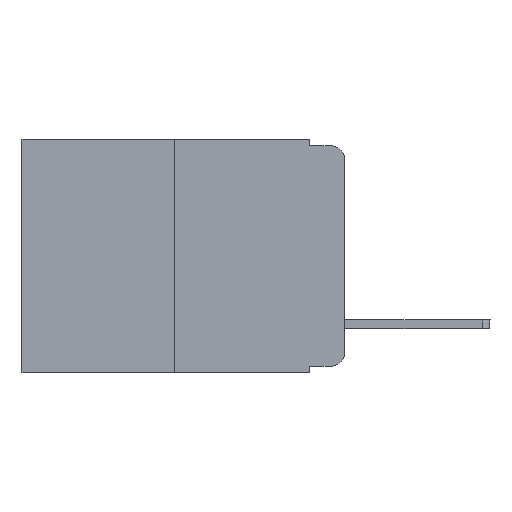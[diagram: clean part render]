
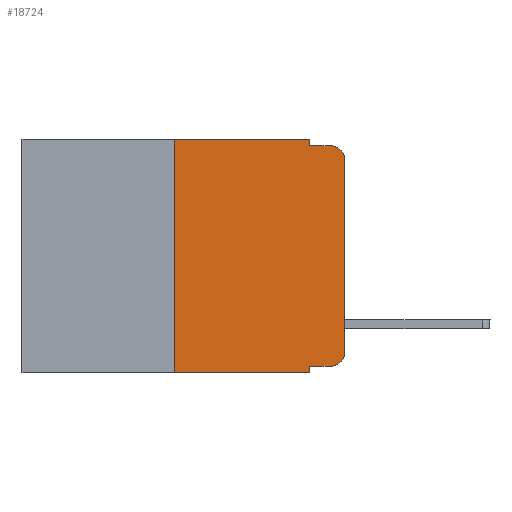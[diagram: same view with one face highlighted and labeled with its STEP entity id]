
A CAD part, left-side view. The second image highlights one B-rep face of the part: STEP entity #18724.
In plain terms, the highlighted planar face has unit normal (-1, 0, 0).
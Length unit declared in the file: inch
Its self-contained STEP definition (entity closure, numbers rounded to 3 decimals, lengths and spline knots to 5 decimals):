
#69 = CARTESIAN_POINT ( 'NONE',  ( 0., 0.473, -0.343 ) ) ;
#344 = EDGE_CURVE ( 'NONE', #3912, #13059, #18565, .T. ) ;
#628 = CARTESIAN_POINT ( 'NONE',  ( 0., 0.473, 0. ) ) ;
#632 = VERTEX_POINT ( 'NONE', #6280 ) ;
#935 = CARTESIAN_POINT ( 'NONE',  ( 0., 0., 0. ) ) ;
#1040 = EDGE_LOOP ( 'NONE', ( #3596, #14313, #4611, #19272, #6123, #4788, #12119, #1695, #17267, #2016 ) ) ;
#1099 = DIRECTION ( 'NONE',  ( 0., 0., -1. ) ) ;
#1208 = LINE ( 'NONE', #7772, #21582 ) ;
#1695 = ORIENTED_EDGE ( 'NONE', *, *, #13113, .F. ) ;
#1750 = VECTOR ( 'NONE', #11619, 39.37008 ) ;
#1966 = CARTESIAN_POINT ( 'NONE',  ( 0., 0., -0.313 ) ) ;
#2016 = ORIENTED_EDGE ( 'NONE', *, *, #19109, .T. ) ;
#2092 = AXIS2_PLACEMENT_3D ( 'NONE', #628, #16011, #15894 ) ;
#2536 = EDGE_CURVE ( 'NONE', #21152, #7386, #18990, .T. ) ;
#3596 = ORIENTED_EDGE ( 'NONE', *, *, #9502, .T. ) ;
#3912 = VERTEX_POINT ( 'NONE', #12076 ) ;
#4255 = AXIS2_PLACEMENT_3D ( 'NONE', #5516, #17437, #12302 ) ;
#4335 = CARTESIAN_POINT ( 'NONE',  ( 0., 0.051, -0.343 ) ) ;
#4606 = CIRCLE ( 'NONE', #4255, 0.02 ) ;
#4611 = ORIENTED_EDGE ( 'NONE', *, *, #344, .F. ) ;
#4696 = VECTOR ( 'NONE', #6855, 39.37008 ) ;
#4788 = ORIENTED_EDGE ( 'NONE', *, *, #8584, .F. ) ;
#4838 = CARTESIAN_POINT ( 'NONE',  ( 0., 0.051, 0. ) ) ;
#5003 = VERTEX_POINT ( 'NONE', #1966 ) ;
#5308 = EDGE_CURVE ( 'NONE', #7377, #13059, #10827, .T. ) ;
#5404 = CARTESIAN_POINT ( 'NONE',  ( 0., 0.051, -0.01 ) ) ;
#5516 = CARTESIAN_POINT ( 'NONE',  ( 0., 0.02, -0.313 ) ) ;
#6123 = ORIENTED_EDGE ( 'NONE', *, *, #12075, .F. ) ;
#6268 = VECTOR ( 'NONE', #18670, 39.37008 ) ;
#6280 = CARTESIAN_POINT ( 'NONE',  ( 0., 0.051, 0. ) ) ;
#6855 = DIRECTION ( 'NONE',  ( 0., -1., 0. ) ) ;
#7026 = CARTESIAN_POINT ( 'NONE',  ( 0., 0.25, 0. ) ) ;
#7368 = CARTESIAN_POINT ( 'NONE',  ( 0., 0.051, -0.333 ) ) ;
#7377 = VERTEX_POINT ( 'NONE', #10889 ) ;
#7386 = VERTEX_POINT ( 'NONE', #4335 ) ;
#7725 = DIRECTION ( 'NONE',  ( 0., 0., 1. ) ) ;
#7772 = CARTESIAN_POINT ( 'NONE',  ( 0., 0.051, 0. ) ) ;
#8191 = DIRECTION ( 'NONE',  ( -1., 0., 0. ) ) ;
#8584 = EDGE_CURVE ( 'NONE', #21152, #20888, #10684, .T. ) ;
#8619 = EDGE_CURVE ( 'NONE', #632, #3912, #1208, .T. ) ;
#8916 = CARTESIAN_POINT ( 'NONE',  ( 0., 0.473, 0. ) ) ;
#9178 = CARTESIAN_POINT ( 'NONE',  ( 0., 0.02, -0.01 ) ) ;
#9213 = VECTOR ( 'NONE', #20862, 39.37008 ) ;
#9441 = VECTOR ( 'NONE', #12349, 39.37008 ) ;
#9502 = EDGE_CURVE ( 'NONE', #5003, #7377, #16208, .T. ) ;
#9856 = CARTESIAN_POINT ( 'NONE',  ( 0., 0.02, -0.03 ) ) ;
#10684 = LINE ( 'NONE', #7026, #9441 ) ;
#10764 = EDGE_CURVE ( 'NONE', #19563, #13970, #18857, .T. ) ;
#10827 = CIRCLE ( 'NONE', #13685, 0.02 ) ;
#10889 = CARTESIAN_POINT ( 'NONE',  ( 0., 0., -0.03 ) ) ;
#10906 = VECTOR ( 'NONE', #7725, 39.37008 ) ;
#11619 = DIRECTION ( 'NONE',  ( 0., 0., -1. ) ) ;
#12075 = EDGE_CURVE ( 'NONE', #20888, #632, #14051, .T. ) ;
#12076 = CARTESIAN_POINT ( 'NONE',  ( 0., 0.051, -0.01 ) ) ;
#12119 = ORIENTED_EDGE ( 'NONE', *, *, #2536, .T. ) ;
#12302 = DIRECTION ( 'NONE',  ( 0., 0., -1. ) ) ;
#12349 = DIRECTION ( 'NONE',  ( 0., 0., 1. ) ) ;
#13059 = VERTEX_POINT ( 'NONE', #9178 ) ;
#13113 = EDGE_CURVE ( 'NONE', #19563, #7386, #13288, .T. ) ;
#13288 = LINE ( 'NONE', #4838, #1750 ) ;
#13685 = AXIS2_PLACEMENT_3D ( 'NONE', #9856, #8191, #18113 ) ;
#13970 = VERTEX_POINT ( 'NONE', #21832 ) ;
#14051 = LINE ( 'NONE', #8916, #9213 ) ;
#14313 = ORIENTED_EDGE ( 'NONE', *, *, #5308, .T. ) ;
#15894 = DIRECTION ( 'NONE',  ( 0., 0., -1. ) ) ;
#16011 = DIRECTION ( 'NONE',  ( 1., 0., 0. ) ) ;
#16208 = LINE ( 'NONE', #935, #10906 ) ;
#17267 = ORIENTED_EDGE ( 'NONE', *, *, #10764, .T. ) ;
#17437 = DIRECTION ( 'NONE',  ( -1., 0., 0. ) ) ;
#17615 = DIRECTION ( 'NONE',  ( 0., -1., 0. ) ) ;
#18113 = DIRECTION ( 'NONE',  ( 0., 0., -1. ) ) ;
#18565 = LINE ( 'NONE', #5404, #6268 ) ;
#18670 = DIRECTION ( 'NONE',  ( 0., -1., 0. ) ) ;
#18724 = ADVANCED_FACE ( 'NONE', ( #20815 ), #19355, .F. ) ;
#18857 = LINE ( 'NONE', #20638, #20228 ) ;
#18990 = LINE ( 'NONE', #69, #4696 ) ;
#19092 = CARTESIAN_POINT ( 'NONE',  ( 0., 0.25, 0. ) ) ;
#19109 = EDGE_CURVE ( 'NONE', #13970, #5003, #4606, .T. ) ;
#19272 = ORIENTED_EDGE ( 'NONE', *, *, #8619, .F. ) ;
#19355 = PLANE ( 'NONE',  #2092 ) ;
#19563 = VERTEX_POINT ( 'NONE', #7368 ) ;
#20228 = VECTOR ( 'NONE', #17615, 39.37008 ) ;
#20638 = CARTESIAN_POINT ( 'NONE',  ( 0., 0.051, -0.333 ) ) ;
#20815 = FACE_OUTER_BOUND ( 'NONE', #1040, .T. ) ;
#20862 = DIRECTION ( 'NONE',  ( 0., -1., 0. ) ) ;
#20888 = VERTEX_POINT ( 'NONE', #19092 ) ;
#21152 = VERTEX_POINT ( 'NONE', #21983 ) ;
#21582 = VECTOR ( 'NONE', #1099, 39.37008 ) ;
#21832 = CARTESIAN_POINT ( 'NONE',  ( 0., 0.02, -0.333 ) ) ;
#21983 = CARTESIAN_POINT ( 'NONE',  ( 0., 0.25, -0.343 ) ) ;
